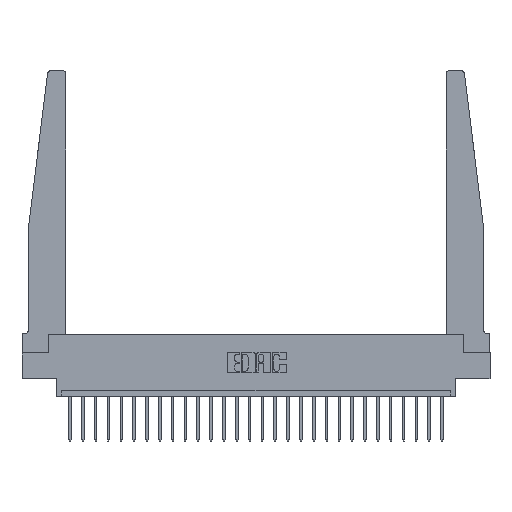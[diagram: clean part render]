
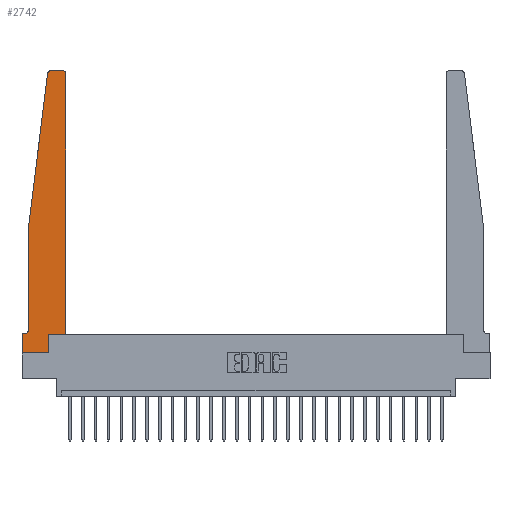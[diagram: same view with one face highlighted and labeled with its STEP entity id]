
A CAD part, top view. The second image highlights one B-rep face of the part: STEP entity #2742.
In plain terms, the highlighted planar face has unit normal (0, 0, 1).
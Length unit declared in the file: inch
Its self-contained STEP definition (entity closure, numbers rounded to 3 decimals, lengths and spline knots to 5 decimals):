
#35 = ORIENTED_EDGE ( 'NONE', *, *, #14570, .T. ) ;
#190 = AXIS2_PLACEMENT_3D ( 'NONE', #13457, #13585, #21482 ) ;
#493 = CIRCLE ( 'NONE', #21980, 0.03 ) ;
#806 = DIRECTION ( 'NONE',  ( 0., 0., 1. ) ) ;
#1010 = ORIENTED_EDGE ( 'NONE', *, *, #20076, .T. ) ;
#1040 = CIRCLE ( 'NONE', #190, 0.03 ) ;
#1191 = PLANE ( 'NONE',  #25252 ) ;
#1332 = VECTOR ( 'NONE', #3910, 39.37008 ) ;
#1372 = EDGE_CURVE ( 'NONE', #13479, #8107, #24736, .T. ) ;
#1427 = EDGE_CURVE ( 'NONE', #5961, #18987, #493, .T. ) ;
#2205 = VERTEX_POINT ( 'NONE', #2567 ) ;
#2359 = LINE ( 'NONE', #15914, #1332 ) ;
#2567 = CARTESIAN_POINT ( 'NONE',  ( 0., 0.1875, 0.37 ) ) ;
#2742 = ADVANCED_FACE ( 'NONE', ( #24615 ), #1191, .T. ) ;
#3820 = CARTESIAN_POINT ( 'NONE',  ( 0., 0., 0.37 ) ) ;
#3900 = DIRECTION ( 'NONE',  ( 1., 0., 0. ) ) ;
#3910 = DIRECTION ( 'NONE',  ( 0., 1., 0. ) ) ;
#4186 = DIRECTION ( 'NONE',  ( -0.122, -0.992, 0. ) ) ;
#4290 = CARTESIAN_POINT ( 'NONE',  ( 0.425, 0.18, 0.37 ) ) ;
#4460 = DIRECTION ( 'NONE',  ( -1., 0., 0. ) ) ;
#4817 = ORIENTED_EDGE ( 'NONE', *, *, #10124, .T. ) ;
#5127 = DIRECTION ( 'NONE',  ( 0., 0., -1. ) ) ;
#5198 = DIRECTION ( 'NONE',  ( 1., 0., 0. ) ) ;
#5367 = LINE ( 'NONE', #3820, #22826 ) ;
#5918 = VECTOR ( 'NONE', #4186, 39.37008 ) ;
#5939 = LINE ( 'NONE', #4290, #11077 ) ;
#5961 = VERTEX_POINT ( 'NONE', #17323 ) ;
#6106 = EDGE_LOOP ( 'NONE', ( #4817, #20516, #35, #13746, #10177, #24367, #24487, #6736, #14370, #1010, #16963, #10753 ) ) ;
#6736 = ORIENTED_EDGE ( 'NONE', *, *, #22315, .T. ) ;
#7144 = DIRECTION ( 'NONE',  ( 1., 0., 0. ) ) ;
#7251 = VECTOR ( 'NONE', #17073, 39.37008 ) ;
#7433 = VERTEX_POINT ( 'NONE', #16780 ) ;
#7505 = LINE ( 'NONE', #25364, #9704 ) ;
#8107 = VERTEX_POINT ( 'NONE', #10149 ) ;
#8820 = CARTESIAN_POINT ( 'NONE',  ( 0.065, 1.25, 0.37 ) ) ;
#8825 = DIRECTION ( 'NONE',  ( 0., 0., 1. ) ) ;
#9071 = CARTESIAN_POINT ( 'NONE',  ( 0., 0.1875, 0.37 ) ) ;
#9131 = CARTESIAN_POINT ( 'NONE',  ( 0.015, 0.2375, 0.37 ) ) ;
#9704 = VECTOR ( 'NONE', #3900, 39.37008 ) ;
#10124 = EDGE_CURVE ( 'NONE', #18987, #17292, #14267, .T. ) ;
#10149 = CARTESIAN_POINT ( 'NONE',  ( 0.065, 0.2375, 0.37 ) ) ;
#10177 = ORIENTED_EDGE ( 'NONE', *, *, #15136, .T. ) ;
#10253 = CARTESIAN_POINT ( 'NONE',  ( 0.065, 1.25, 0.37 ) ) ;
#10753 = ORIENTED_EDGE ( 'NONE', *, *, #1427, .T. ) ;
#11077 = VECTOR ( 'NONE', #13832, 39.37008 ) ;
#11283 = EDGE_CURVE ( 'NONE', #2205, #24060, #5367, .T. ) ;
#11685 = VECTOR ( 'NONE', #20714, 39.37008 ) ;
#11782 = EDGE_CURVE ( 'NONE', #7433, #14388, #2359, .T. ) ;
#12540 = CARTESIAN_POINT ( 'NONE',  ( 0.065, 1.25, 0.37 ) ) ;
#12769 = DIRECTION ( 'NONE',  ( -1., 0., 0. ) ) ;
#13250 = DIRECTION ( 'NONE',  ( 0., -1., 0. ) ) ;
#13457 = CARTESIAN_POINT ( 'NONE',  ( 0.27653, 2.72, 0.37 ) ) ;
#13479 = VERTEX_POINT ( 'NONE', #12540 ) ;
#13585 = DIRECTION ( 'NONE',  ( 0., 0., 1. ) ) ;
#13746 = ORIENTED_EDGE ( 'NONE', *, *, #1372, .T. ) ;
#13832 = DIRECTION ( 'NONE',  ( 0., 1., 0. ) ) ;
#13936 = CARTESIAN_POINT ( 'NONE',  ( 0.425, 0.18, 0.37 ) ) ;
#14267 = LINE ( 'NONE', #23588, #19230 ) ;
#14370 = ORIENTED_EDGE ( 'NONE', *, *, #11782, .T. ) ;
#14388 = VERTEX_POINT ( 'NONE', #15169 ) ;
#14570 = EDGE_CURVE ( 'NONE', #23196, #13479, #17619, .T. ) ;
#15018 = CARTESIAN_POINT ( 'NONE',  ( 0.395, 2.72, 0.37 ) ) ;
#15136 = EDGE_CURVE ( 'NONE', #8107, #15881, #20410, .T. ) ;
#15169 = CARTESIAN_POINT ( 'NONE',  ( 0.2605, 0.18, 0.37 ) ) ;
#15693 = LINE ( 'NONE', #17136, #18896 ) ;
#15881 = VERTEX_POINT ( 'NONE', #22665 ) ;
#15914 = CARTESIAN_POINT ( 'NONE',  ( 0.2605, 0.18, 0.37 ) ) ;
#16780 = CARTESIAN_POINT ( 'NONE',  ( 0.2605, 0., 0.37 ) ) ;
#16963 = ORIENTED_EDGE ( 'NONE', *, *, #25107, .T. ) ;
#17073 = DIRECTION ( 'NONE',  ( 1., 0., 0. ) ) ;
#17136 = CARTESIAN_POINT ( 'NONE',  ( 0.065, 0.1875, 0.37 ) ) ;
#17292 = VERTEX_POINT ( 'NONE', #22370 ) ;
#17323 = CARTESIAN_POINT ( 'NONE',  ( 0.425, 2.72, 0.37 ) ) ;
#17619 = LINE ( 'NONE', #10253, #5918 ) ;
#17668 = CARTESIAN_POINT ( 'NONE',  ( 0., 0., 0.37 ) ) ;
#18896 = VECTOR ( 'NONE', #23333, 39.37008 ) ;
#18944 = CARTESIAN_POINT ( 'NONE',  ( 0.24675, 2.72367, 0.37 ) ) ;
#18987 = VERTEX_POINT ( 'NONE', #19201 ) ;
#19201 = CARTESIAN_POINT ( 'NONE',  ( 0.395, 2.75, 0.37 ) ) ;
#19230 = VECTOR ( 'NONE', #4460, 39.37008 ) ;
#20076 = EDGE_CURVE ( 'NONE', #14388, #25433, #7505, .T. ) ;
#20138 = EDGE_CURVE ( 'NONE', #17292, #23196, #1040, .T. ) ;
#20410 = CIRCLE ( 'NONE', #21644, 0.05 ) ;
#20516 = ORIENTED_EDGE ( 'NONE', *, *, #20138, .T. ) ;
#20714 = DIRECTION ( 'NONE',  ( 0., -1., 0. ) ) ;
#21482 = DIRECTION ( 'NONE',  ( 1., 0., 0. ) ) ;
#21644 = AXIS2_PLACEMENT_3D ( 'NONE', #9131, #5127, #12769 ) ;
#21980 = AXIS2_PLACEMENT_3D ( 'NONE', #15018, #806, #5198 ) ;
#22315 = EDGE_CURVE ( 'NONE', #24060, #7433, #24590, .T. ) ;
#22370 = CARTESIAN_POINT ( 'NONE',  ( 0.27653, 2.75, 0.37 ) ) ;
#22513 = CARTESIAN_POINT ( 'NONE',  ( 0., 0., 0.37 ) ) ;
#22665 = CARTESIAN_POINT ( 'NONE',  ( 0.015, 0.1875, 0.37 ) ) ;
#22826 = VECTOR ( 'NONE', #13250, 39.37008 ) ;
#23196 = VERTEX_POINT ( 'NONE', #18944 ) ;
#23333 = DIRECTION ( 'NONE',  ( -1., 0., 0. ) ) ;
#23588 = CARTESIAN_POINT ( 'NONE',  ( 0.25, 2.75, 0.37 ) ) ;
#24060 = VERTEX_POINT ( 'NONE', #17668 ) ;
#24367 = ORIENTED_EDGE ( 'NONE', *, *, #24513, .T. ) ;
#24487 = ORIENTED_EDGE ( 'NONE', *, *, #11283, .T. ) ;
#24513 = EDGE_CURVE ( 'NONE', #15881, #2205, #15693, .T. ) ;
#24590 = LINE ( 'NONE', #22513, #7251 ) ;
#24615 = FACE_OUTER_BOUND ( 'NONE', #6106, .T. ) ;
#24736 = LINE ( 'NONE', #8820, #11685 ) ;
#25107 = EDGE_CURVE ( 'NONE', #25433, #5961, #5939, .T. ) ;
#25252 = AXIS2_PLACEMENT_3D ( 'NONE', #9071, #8825, #7144 ) ;
#25364 = CARTESIAN_POINT ( 'NONE',  ( 0.425, 0.18, 0.37 ) ) ;
#25433 = VERTEX_POINT ( 'NONE', #13936 ) ;
